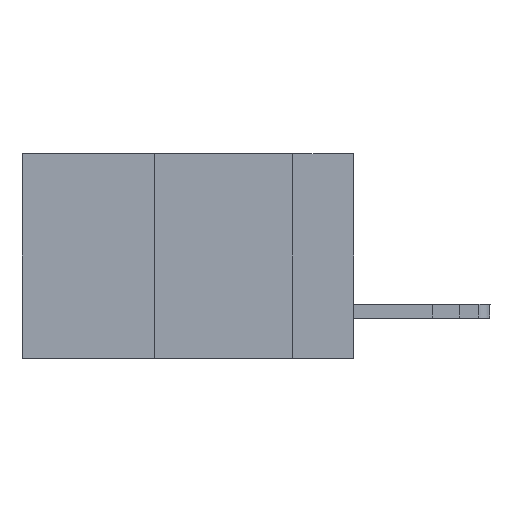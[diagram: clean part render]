
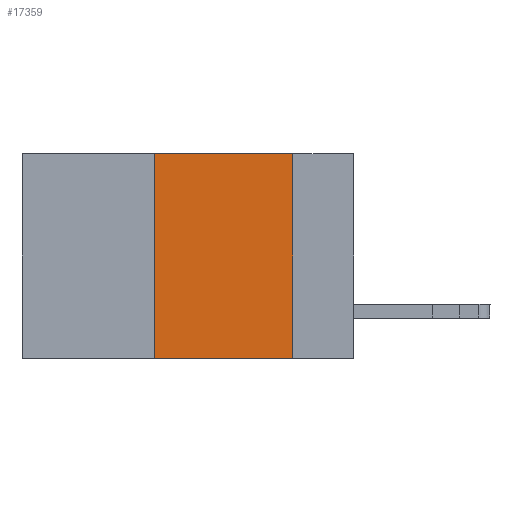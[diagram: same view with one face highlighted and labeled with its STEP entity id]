
A CAD part, left-side view. The second image highlights one B-rep face of the part: STEP entity #17359.
In plain terms, the highlighted planar face has unit normal (-1, 0, 0).
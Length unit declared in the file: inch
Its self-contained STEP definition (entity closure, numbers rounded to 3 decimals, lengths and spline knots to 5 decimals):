
#31 = CARTESIAN_POINT ( 'NONE',  ( 0., 0.11, -0.37 ) ) ;
#613 = EDGE_CURVE ( 'NONE', #8519, #7231, #7755, .T. ) ;
#1024 = VECTOR ( 'NONE', #7754, 39.37008 ) ;
#1230 = EDGE_CURVE ( 'NONE', #7231, #7916, #6808, .T. ) ;
#2023 = EDGE_LOOP ( 'NONE', ( #18197, #16761, #18630, #3835 ) ) ;
#3348 = VERTEX_POINT ( 'NONE', #31 ) ;
#3835 = ORIENTED_EDGE ( 'NONE', *, *, #16286, .T. ) ;
#4593 = VECTOR ( 'NONE', #7220, 39.37008 ) ;
#5050 = DIRECTION ( 'NONE',  ( 1., 0., 0. ) ) ;
#6080 = CARTESIAN_POINT ( 'NONE',  ( 0., 0.36, 0. ) ) ;
#6808 = LINE ( 'NONE', #7450, #9760 ) ;
#7220 = DIRECTION ( 'NONE',  ( 0., 0., 1. ) ) ;
#7231 = VERTEX_POINT ( 'NONE', #6080 ) ;
#7450 = CARTESIAN_POINT ( 'NONE',  ( 0., 0.6, 0. ) ) ;
#7630 = CARTESIAN_POINT ( 'NONE',  ( 0., 0.11, 0. ) ) ;
#7748 = EDGE_CURVE ( 'NONE', #7916, #3348, #16381, .T. ) ;
#7754 = DIRECTION ( 'NONE',  ( 0., 0., -1. ) ) ;
#7755 = LINE ( 'NONE', #13169, #4593 ) ;
#7916 = VERTEX_POINT ( 'NONE', #10519 ) ;
#8519 = VERTEX_POINT ( 'NONE', #12738 ) ;
#9760 = VECTOR ( 'NONE', #11758, 39.37008 ) ;
#10027 = DIRECTION ( 'NONE',  ( 0., -1., 0. ) ) ;
#10153 = CARTESIAN_POINT ( 'NONE',  ( 0., 0.6, -0.37 ) ) ;
#10519 = CARTESIAN_POINT ( 'NONE',  ( 0., 0.11, 0. ) ) ;
#10678 = LINE ( 'NONE', #10153, #13181 ) ;
#11758 = DIRECTION ( 'NONE',  ( 0., -1., 0. ) ) ;
#12102 = FACE_OUTER_BOUND ( 'NONE', #2023, .T. ) ;
#12738 = CARTESIAN_POINT ( 'NONE',  ( 0., 0.36, -0.37 ) ) ;
#13169 = CARTESIAN_POINT ( 'NONE',  ( 0., 0.36, 0. ) ) ;
#13181 = VECTOR ( 'NONE', #10027, 39.37008 ) ;
#13673 = PLANE ( 'NONE',  #18281 ) ;
#15108 = CARTESIAN_POINT ( 'NONE',  ( 0., 0.6, 0. ) ) ;
#15547 = DIRECTION ( 'NONE',  ( 0., 0., -1. ) ) ;
#16286 = EDGE_CURVE ( 'NONE', #8519, #3348, #10678, .T. ) ;
#16381 = LINE ( 'NONE', #7630, #1024 ) ;
#16761 = ORIENTED_EDGE ( 'NONE', *, *, #1230, .F. ) ;
#17359 = ADVANCED_FACE ( 'NONE', ( #12102 ), #13673, .F. ) ;
#18197 = ORIENTED_EDGE ( 'NONE', *, *, #7748, .F. ) ;
#18281 = AXIS2_PLACEMENT_3D ( 'NONE', #15108, #5050, #15547 ) ;
#18630 = ORIENTED_EDGE ( 'NONE', *, *, #613, .F. ) ;
